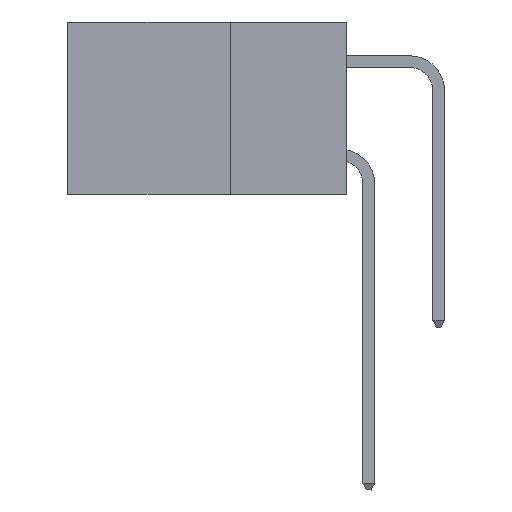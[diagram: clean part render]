
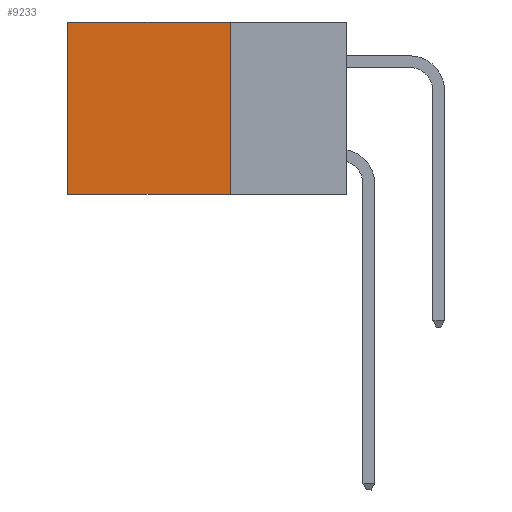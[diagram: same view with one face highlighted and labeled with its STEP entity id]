
A CAD part, left-side view. The second image highlights one B-rep face of the part: STEP entity #9233.
In plain terms, the highlighted planar face has unit normal (-1, 0, 0).
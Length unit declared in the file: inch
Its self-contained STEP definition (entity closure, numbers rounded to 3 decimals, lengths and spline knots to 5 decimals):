
#452 = ORIENTED_EDGE ( 'NONE', *, *, #9272, .T. ) ;
#689 = VERTEX_POINT ( 'NONE', #5045 ) ;
#784 = ORIENTED_EDGE ( 'NONE', *, *, #8778, .F. ) ;
#1526 = EDGE_LOOP ( 'NONE', ( #452, #11953, #784, #5385 ) ) ;
#1698 = CARTESIAN_POINT ( 'NONE',  ( 0.2875, 0.25, 0. ) ) ;
#1949 = DIRECTION ( 'NONE',  ( 0., 0., -1. ) ) ;
#2826 = FACE_OUTER_BOUND ( 'NONE', #1526, .T. ) ;
#2894 = VECTOR ( 'NONE', #1949, 39.37008 ) ;
#2945 = DIRECTION ( 'NONE',  ( 0., 1., 0. ) ) ;
#3206 = VERTEX_POINT ( 'NONE', #11267 ) ;
#3646 = CARTESIAN_POINT ( 'NONE',  ( 0.2875, 0.25, 0. ) ) ;
#3945 = CARTESIAN_POINT ( 'NONE',  ( 0.2875, 0.25, -0.37 ) ) ;
#4570 = LINE ( 'NONE', #3646, #6836 ) ;
#4628 = DIRECTION ( 'NONE',  ( 1., 0., 0. ) ) ;
#5045 = CARTESIAN_POINT ( 'NONE',  ( 0.2875, 0.6, -0.37 ) ) ;
#5385 = ORIENTED_EDGE ( 'NONE', *, *, #9249, .T. ) ;
#5556 = CARTESIAN_POINT ( 'NONE',  ( 0.2875, 0.25, 0. ) ) ;
#6050 = LINE ( 'NONE', #3945, #6670 ) ;
#6258 = VECTOR ( 'NONE', #6675, 39.37008 ) ;
#6552 = LINE ( 'NONE', #10350, #2894 ) ;
#6670 = VECTOR ( 'NONE', #2945, 39.37008 ) ;
#6675 = DIRECTION ( 'NONE',  ( 0., 1., 0. ) ) ;
#6766 = VERTEX_POINT ( 'NONE', #8879 ) ;
#6836 = VECTOR ( 'NONE', #11233, 39.37008 ) ;
#8778 = EDGE_CURVE ( 'NONE', #3206, #6766, #4570, .T. ) ;
#8850 = CARTESIAN_POINT ( 'NONE',  ( 0.2875, 0.6, 0. ) ) ;
#8879 = CARTESIAN_POINT ( 'NONE',  ( 0.2875, 0.25, -0.37 ) ) ;
#9233 = ADVANCED_FACE ( 'NONE', ( #2826 ), #10287, .F. ) ;
#9249 = EDGE_CURVE ( 'NONE', #3206, #11237, #9471, .T. ) ;
#9272 = EDGE_CURVE ( 'NONE', #11237, #689, #6552, .T. ) ;
#9384 = EDGE_CURVE ( 'NONE', #6766, #689, #6050, .T. ) ;
#9418 = DIRECTION ( 'NONE',  ( 0., 0., -1. ) ) ;
#9471 = LINE ( 'NONE', #5556, #6258 ) ;
#10287 = PLANE ( 'NONE',  #10630 ) ;
#10350 = CARTESIAN_POINT ( 'NONE',  ( 0.2875, 0.6, 0. ) ) ;
#10630 = AXIS2_PLACEMENT_3D ( 'NONE', #1698, #4628, #9418 ) ;
#11233 = DIRECTION ( 'NONE',  ( 0., 0., -1. ) ) ;
#11237 = VERTEX_POINT ( 'NONE', #8850 ) ;
#11267 = CARTESIAN_POINT ( 'NONE',  ( 0.2875, 0.25, 0. ) ) ;
#11953 = ORIENTED_EDGE ( 'NONE', *, *, #9384, .F. ) ;
